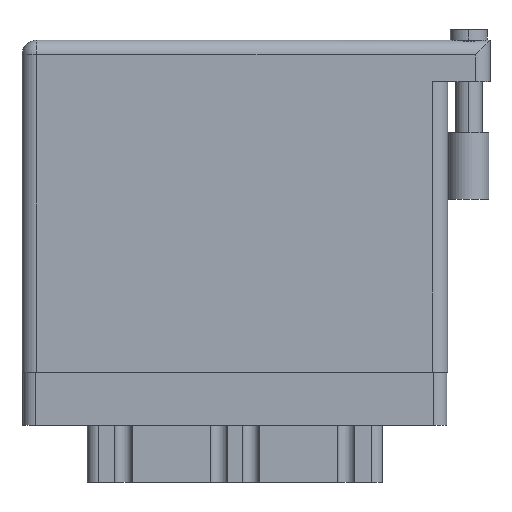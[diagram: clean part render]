
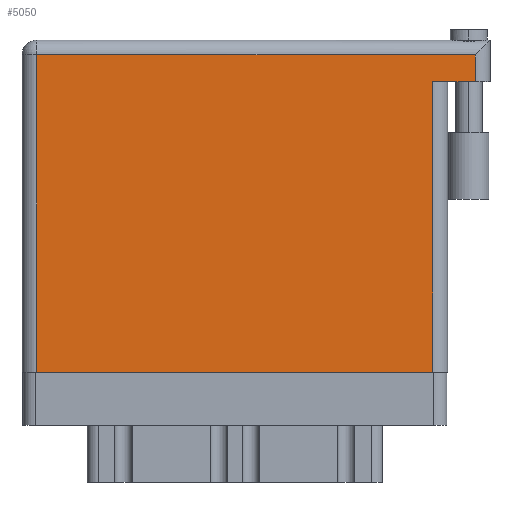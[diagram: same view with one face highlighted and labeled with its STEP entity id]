
A CAD part, front view. The second image highlights one B-rep face of the part: STEP entity #5050.
In plain terms, the highlighted face is planar.
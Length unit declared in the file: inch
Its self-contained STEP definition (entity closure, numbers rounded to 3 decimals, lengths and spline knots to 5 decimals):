
#429 = VERTEX_POINT ( 'NONE', #6376 ) ;
#634 = EDGE_CURVE ( 'NONE', #10332, #23034, #37861, .T. ) ;
#1177 = FACE_OUTER_BOUND ( 'NONE', #30145, .T. ) ;
#1823 = CARTESIAN_POINT ( 'NONE',  ( 0., 1.496, 0. ) ) ;
#2000 = CARTESIAN_POINT ( 'NONE',  ( 1.938, 0., 0. ) ) ;
#2551 = DIRECTION ( 'NONE',  ( 1., 0., 0. ) ) ;
#2760 = EDGE_CURVE ( 'NONE', #23034, #23537, #8011, .T. ) ;
#3455 = EDGE_CURVE ( 'NONE', #429, #7984, #23917, .T. ) ;
#4281 = DIRECTION ( 'NONE',  ( -1., 0., 0. ) ) ;
#4573 = VECTOR ( 'NONE', #21219, 39.37008 ) ;
#5050 = ADVANCED_FACE ( 'NONE', ( #1177 ), #24111, .F. ) ;
#6376 = CARTESIAN_POINT ( 'NONE',  ( 0.07, 0., 0. ) ) ;
#7125 = LINE ( 'NONE', #31743, #28191 ) ;
#7459 = CARTESIAN_POINT ( 'NONE',  ( 0.07, 1.496, 0. ) ) ;
#7984 = VERTEX_POINT ( 'NONE', #2000 ) ;
#8011 = LINE ( 'NONE', #1823, #30527 ) ;
#8658 = VECTOR ( 'NONE', #11010, 39.37008 ) ;
#8834 = DIRECTION ( 'NONE',  ( -1., 0., 0. ) ) ;
#9113 = CARTESIAN_POINT ( 'NONE',  ( 0., 0., 0. ) ) ;
#10332 = VERTEX_POINT ( 'NONE', #37193 ) ;
#10512 = AXIS2_PLACEMENT_3D ( 'NONE', #21972, #24687, #4281 ) ;
#11010 = DIRECTION ( 'NONE',  ( 0., 1., 0. ) ) ;
#15568 = ORIENTED_EDGE ( 'NONE', *, *, #2760, .T. ) ;
#15802 = LINE ( 'NONE', #24542, #4573 ) ;
#15885 = EDGE_CURVE ( 'NONE', #7984, #38008, #15802, .T. ) ;
#16849 = CARTESIAN_POINT ( 'NONE',  ( 2.138, 1.566, 0. ) ) ;
#18988 = DIRECTION ( 'NONE',  ( 0., -1., 0. ) ) ;
#19552 = EDGE_CURVE ( 'NONE', #10332, #38008, #35480, .T. ) ;
#19626 = ORIENTED_EDGE ( 'NONE', *, *, #19552, .F. ) ;
#20068 = DIRECTION ( 'NONE',  ( -1., 0., 0. ) ) ;
#21196 = EDGE_CURVE ( 'NONE', #23537, #429, #7125, .T. ) ;
#21219 = DIRECTION ( 'NONE',  ( 0., 1., 0. ) ) ;
#21888 = ORIENTED_EDGE ( 'NONE', *, *, #15885, .T. ) ;
#21972 = CARTESIAN_POINT ( 'NONE',  ( 0., 1.566, 0. ) ) ;
#23034 = VERTEX_POINT ( 'NONE', #29047 ) ;
#23258 = CARTESIAN_POINT ( 'NONE',  ( 2.208, 1.369, 0. ) ) ;
#23537 = VERTEX_POINT ( 'NONE', #7459 ) ;
#23917 = LINE ( 'NONE', #9113, #33650 ) ;
#24111 = PLANE ( 'NONE',  #10512 ) ;
#24542 = CARTESIAN_POINT ( 'NONE',  ( 1.938, 1.369, 0. ) ) ;
#24687 = DIRECTION ( 'NONE',  ( 0., 0., -1. ) ) ;
#25697 = VECTOR ( 'NONE', #8834, 39.37008 ) ;
#28191 = VECTOR ( 'NONE', #18988, 39.37008 ) ;
#29047 = CARTESIAN_POINT ( 'NONE',  ( 2.138, 1.496, 0. ) ) ;
#30145 = EDGE_LOOP ( 'NONE', ( #31909, #21888, #19626, #38294, #15568, #33372 ) ) ;
#30527 = VECTOR ( 'NONE', #20068, 39.37008 ) ;
#31743 = CARTESIAN_POINT ( 'NONE',  ( 0.07, 0., 0. ) ) ;
#31909 = ORIENTED_EDGE ( 'NONE', *, *, #3455, .T. ) ;
#33372 = ORIENTED_EDGE ( 'NONE', *, *, #21196, .T. ) ;
#33650 = VECTOR ( 'NONE', #2551, 39.37008 ) ;
#35480 = LINE ( 'NONE', #23258, #25697 ) ;
#37193 = CARTESIAN_POINT ( 'NONE',  ( 2.138, 1.369, 0. ) ) ;
#37861 = LINE ( 'NONE', #16849, #8658 ) ;
#38008 = VERTEX_POINT ( 'NONE', #38269 ) ;
#38269 = CARTESIAN_POINT ( 'NONE',  ( 1.938, 1.369, 0. ) ) ;
#38294 = ORIENTED_EDGE ( 'NONE', *, *, #634, .T. ) ;
